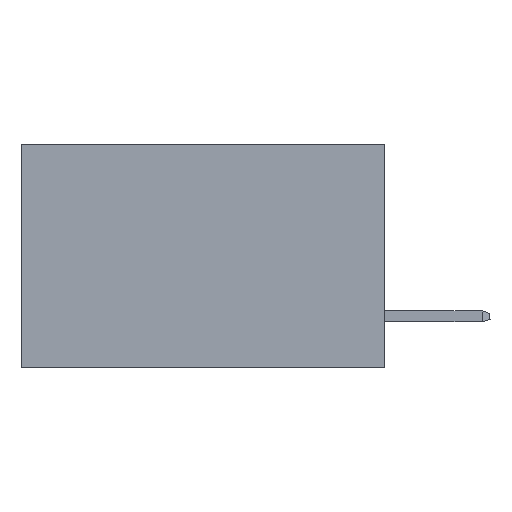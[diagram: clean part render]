
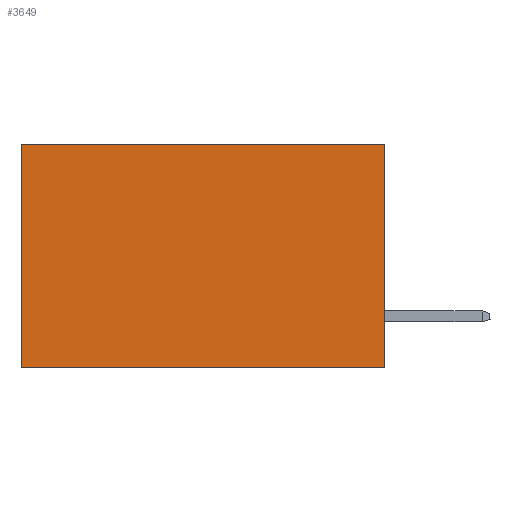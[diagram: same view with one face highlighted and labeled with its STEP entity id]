
A CAD part, left-side view. The second image highlights one B-rep face of the part: STEP entity #3649.
In plain terms, the highlighted planar face has unit normal (-1, 0, 0).
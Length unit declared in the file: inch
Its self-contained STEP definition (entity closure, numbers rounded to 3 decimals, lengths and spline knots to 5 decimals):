
#46 = FACE_OUTER_BOUND ( 'NONE', #623, .T. ) ;
#402 = LINE ( 'NONE', #7829, #4664 ) ;
#427 = EDGE_CURVE ( 'NONE', #7572, #6221, #835, .T. ) ;
#584 = EDGE_CURVE ( 'NONE', #6221, #8954, #402, .T. ) ;
#623 = EDGE_LOOP ( 'NONE', ( #2474, #2468, #2442, #5291 ) ) ;
#835 = LINE ( 'NONE', #4667, #5026 ) ;
#1619 = CARTESIAN_POINT ( 'NONE',  ( 0.298, 0., -0.37 ) ) ;
#1738 = DIRECTION ( 'NONE',  ( 0., 0., -1. ) ) ;
#1800 = EDGE_CURVE ( 'NONE', #6304, #8954, #3602, .T. ) ;
#1821 = EDGE_CURVE ( 'NONE', #7572, #6304, #5431, .T. ) ;
#2178 = CARTESIAN_POINT ( 'NONE',  ( 0.298, 0., 0. ) ) ;
#2442 = ORIENTED_EDGE ( 'NONE', *, *, #1821, .F. ) ;
#2468 = ORIENTED_EDGE ( 'NONE', *, *, #1800, .F. ) ;
#2474 = ORIENTED_EDGE ( 'NONE', *, *, #584, .T. ) ;
#2796 = DIRECTION ( 'NONE',  ( 0., 1., 0. ) ) ;
#3425 = CARTESIAN_POINT ( 'NONE',  ( 0.298, 0.6, -0.37 ) ) ;
#3602 = LINE ( 'NONE', #1619, #7239 ) ;
#3649 = ADVANCED_FACE ( 'NONE', ( #46 ), #5335, .F. ) ;
#4241 = DIRECTION ( 'NONE',  ( 0., 0., -1. ) ) ;
#4625 = CARTESIAN_POINT ( 'NONE',  ( 0.298, 0., 0. ) ) ;
#4664 = VECTOR ( 'NONE', #8343, 39.37008 ) ;
#4667 = CARTESIAN_POINT ( 'NONE',  ( 0.298, 0., 0. ) ) ;
#5000 = CARTESIAN_POINT ( 'NONE',  ( 0.298, 0., -0.37 ) ) ;
#5026 = VECTOR ( 'NONE', #2796, 39.37008 ) ;
#5291 = ORIENTED_EDGE ( 'NONE', *, *, #427, .T. ) ;
#5335 = PLANE ( 'NONE',  #7028 ) ;
#5431 = LINE ( 'NONE', #5902, #6834 ) ;
#5696 = CARTESIAN_POINT ( 'NONE',  ( 0.298, 0.6, 0. ) ) ;
#5902 = CARTESIAN_POINT ( 'NONE',  ( 0.298, 0., 0. ) ) ;
#6221 = VERTEX_POINT ( 'NONE', #5696 ) ;
#6304 = VERTEX_POINT ( 'NONE', #5000 ) ;
#6834 = VECTOR ( 'NONE', #1738, 39.37008 ) ;
#7028 = AXIS2_PLACEMENT_3D ( 'NONE', #4625, #8691, #4241 ) ;
#7239 = VECTOR ( 'NONE', #7985, 39.37008 ) ;
#7572 = VERTEX_POINT ( 'NONE', #2178 ) ;
#7829 = CARTESIAN_POINT ( 'NONE',  ( 0.298, 0.6, 0. ) ) ;
#7985 = DIRECTION ( 'NONE',  ( 0., 1., 0. ) ) ;
#8343 = DIRECTION ( 'NONE',  ( 0., 0., -1. ) ) ;
#8691 = DIRECTION ( 'NONE',  ( 1., 0., 0. ) ) ;
#8954 = VERTEX_POINT ( 'NONE', #3425 ) ;
